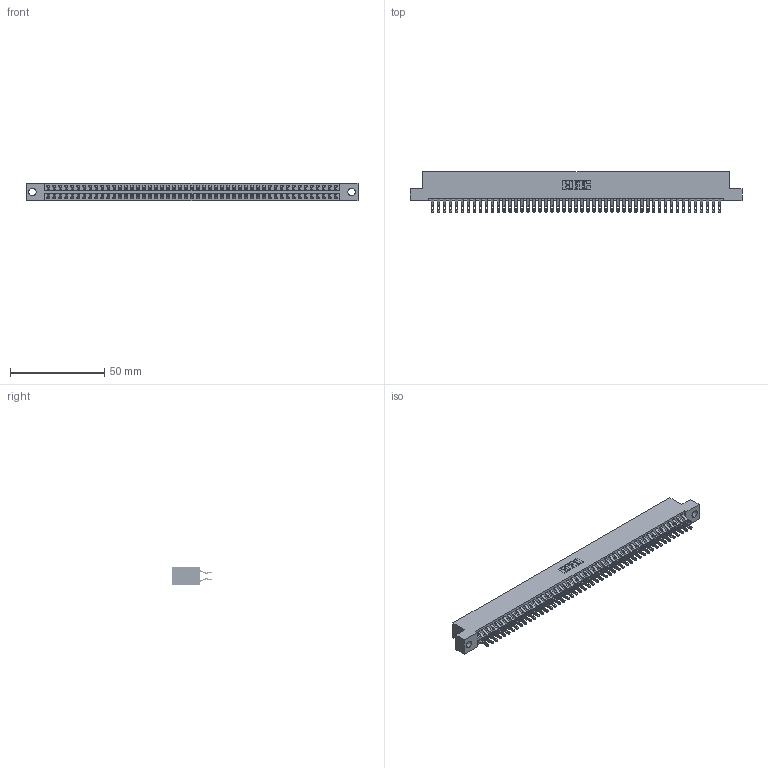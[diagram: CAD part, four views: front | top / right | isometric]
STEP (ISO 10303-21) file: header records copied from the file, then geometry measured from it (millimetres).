
FILE_DESCRIPTION (( 'STEP AP203' ), '1' );
FILE_NAME ('396-098-555-204.STEP', '2019-10-31T05:04:46', ( '' ), ( '' ), 'SwSTEP 2.0', 'SolidWorks 2016', '' );
FILE_SCHEMA (( 'CONFIG_CONTROL_DESIGN' ));
Length unit declared in the file: inch
Products named in the file (3): 396-098-555-204; 346 Part_Flush Mounting Lugs - 0.156 Dia-TH; 345-292-001_555 Tail
Assembly tree (99 placements, depth 2):
  396-098-555-204
    346 Part_Flush Mounting Lugs - 0.156 Dia-TH
    345-292-001_555 Tail  x98
Bounding box: 176.15 x 21.46 x 9.4 mm (x, y, z)
Volume: 17427.5 mm3; surface area: 24891.9 mm2
Topology: 99 solids, 99 shells, 5806 faces, 18263 edges, 12174 vertices
Faces by surface type: plane 3310, cylinder 2496
Entity records: 31365 total; most frequent: CARTESIAN_POINT 5194, ORIENTED_EDGE 5098, DIRECTION 4597, EDGE_CURVE 2549, LINE 2201, VECTOR 2201, VERTEX_POINT 1698, AXIS2_PLACEMENT_3D 1198
